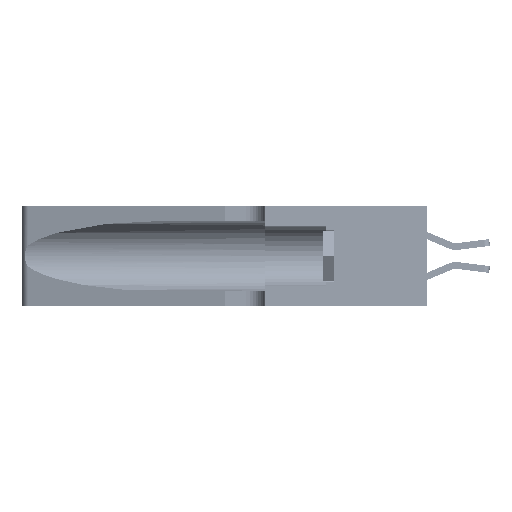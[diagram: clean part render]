
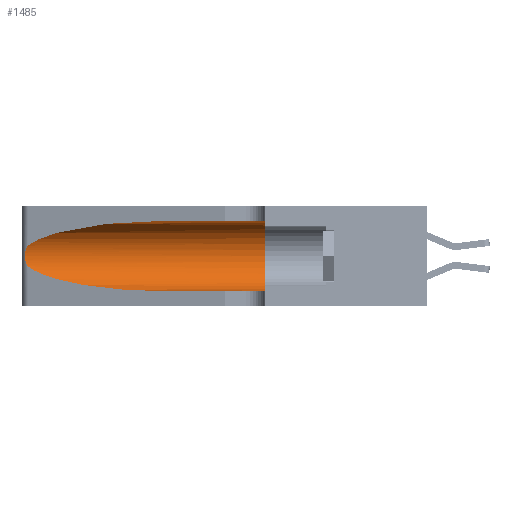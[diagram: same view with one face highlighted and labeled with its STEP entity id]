
A CAD part, left-side view. The second image highlights one B-rep face of the part: STEP entity #1485.
In plain terms, the highlighted cylindrical face has radius 3.308 mm (diameter 6.617 mm), a partial arc.
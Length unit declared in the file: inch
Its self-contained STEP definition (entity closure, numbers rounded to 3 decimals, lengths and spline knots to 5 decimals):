
#673 = ORIENTED_EDGE ( 'NONE', *, *, #36056, .T. ) ;
#773 = EDGE_LOOP ( 'NONE', ( #33767, #15607, #46806, #673, #40579, #41703 ) ) ;
#1485 = ADVANCED_FACE ( 'NONE', ( #13631 ), #41442, .F. ) ;
#1760 = DIRECTION ( 'NONE',  ( 0., -1., 0. ) ) ;
#2161 = VERTEX_POINT ( 'NONE', #34714 ) ;
#2343 = CARTESIAN_POINT ( 'NONE',  ( 0.18966, 0.96281, 0.31525 ) ) ;
#3633 = CARTESIAN_POINT ( 'NONE',  ( 0.25787, 1.23484, 0.2124 ) ) ;
#4534 = CARTESIAN_POINT ( 'NONE',  ( 0.25487, 1.22718, 0.14631 ) ) ;
#4576 = VERTEX_POINT ( 'NONE', #5747 ) ;
#5747 = CARTESIAN_POINT ( 'NONE',  ( 0.25487, 1.22718, 0.14631 ) ) ;
#7349 = CARTESIAN_POINT ( 'NONE',  ( 0.26018, 1.23835, 0.19895 ) ) ;
#8048 = CARTESIAN_POINT ( 'NONE',  ( 0.1305, 0.35, 0.05475 ) ) ;
#8570 = CARTESIAN_POINT ( 'NONE',  ( 0.25487, 1.22718, 0.22369 ) ) ;
#9151 = CARTESIAN_POINT ( 'NONE',  ( 0.1305, 1.61858, 0.185 ) ) ;
#10174 = EDGE_CURVE ( 'NONE', #12046, #4576, #31146, .T. ) ;
#10722 =( BOUNDED_CURVE ( )  B_SPLINE_CURVE ( 3, ( #4534, #33698, #11895, #37339 ),
 .UNSPECIFIED., .F., .T. ) 
 B_SPLINE_CURVE_WITH_KNOTS ( ( 4, 4 ),
 ( 3.44316, 4.71239 ),
 .UNSPECIFIED. ) 
 CURVE ( )  GEOMETRIC_REPRESENTATION_ITEM ( )  RATIONAL_B_SPLINE_CURVE ( ( 1., 0.87, 0.87, 1. ) ) 
 REPRESENTATION_ITEM ( '' )  );
#11016 = CARTESIAN_POINT ( 'NONE',  ( 0.26075, 1.23896, 0.178 ) ) ;
#11130 = CARTESIAN_POINT ( 'NONE',  ( 0.1305, 1.61858, 0.05475 ) ) ;
#11132 = AXIS2_PLACEMENT_3D ( 'NONE', #9151, #1760, #34617 ) ;
#11193 = DIRECTION ( 'NONE',  ( 0., -1., 0. ) ) ;
#11451 = AXIS2_PLACEMENT_3D ( 'NONE', #42541, #20803, #46184 ) ;
#11895 = CARTESIAN_POINT ( 'NONE',  ( 0.18966, 0.96281, 0.05475 ) ) ;
#12046 = VERTEX_POINT ( 'NONE', #8570 ) ;
#12978 = CARTESIAN_POINT ( 'NONE',  ( 0.1305, 0.72297, 0.31525 ) ) ;
#13415 = CARTESIAN_POINT ( 'NONE',  ( 0.25487, 1.22718, 0.22369 ) ) ;
#13631 = FACE_OUTER_BOUND ( 'NONE', #773, .T. ) ;
#14721 = CARTESIAN_POINT ( 'NONE',  ( 0.25856, 1.23593, 0.16098 ) ) ;
#15607 = ORIENTED_EDGE ( 'NONE', *, *, #10174, .T. ) ;
#18196 = CARTESIAN_POINT ( 'NONE',  ( 0.25487, 1.22718, 0.22369 ) ) ;
#18344 = CARTESIAN_POINT ( 'NONE',  ( 0.25639, 1.23186, 0.15144 ) ) ;
#20803 = DIRECTION ( 'NONE',  ( 0., 1., 0. ) ) ;
#21491 = CARTESIAN_POINT ( 'NONE',  ( 0.1305, 0.72297, 0.05475 ) ) ;
#22017 = CARTESIAN_POINT ( 'NONE',  ( 0.25487, 1.22718, 0.14631 ) ) ;
#25516 = CARTESIAN_POINT ( 'NONE',  ( 0.25639, 1.23184, 0.21858 ) ) ;
#26188 = VECTOR ( 'NONE', #11193, 39.37008 ) ;
#27868 = CARTESIAN_POINT ( 'NONE',  ( 0.1305, 0.72297, 0.31525 ) ) ;
#27886 = VERTEX_POINT ( 'NONE', #21491 ) ;
#28393 = EDGE_CURVE ( 'NONE', #2161, #38940, #32527, .T. ) ;
#29145 = CARTESIAN_POINT ( 'NONE',  ( 0.25854, 1.2359, 0.20912 ) ) ;
#31146 = B_SPLINE_CURVE_WITH_KNOTS ( 'NONE', 3,
 ( #18196, #36307, #25516, #3633, #29145, #7349, #32823, #11016, #36464, #14721, #40090, #18344, #43733, #22017 ),
 .UNSPECIFIED., .F., .F.,
 ( 4, 2, 2, 2, 2, 2, 4 ),
 ( 0., 0.00027, 0.00053, 0.00107, 0.0016, 0.00187, 0.00214 ),
 .UNSPECIFIED. ) ;
#31334 = VERTEX_POINT ( 'NONE', #12978 ) ;
#32527 = CIRCLE ( 'NONE', #11451, 0.13025 ) ;
#32615 =( BOUNDED_CURVE ( )  B_SPLINE_CURVE ( 3, ( #27868, #2343, #35198, #13415 ),
 .UNSPECIFIED., .F., .F. ) 
 B_SPLINE_CURVE_WITH_KNOTS ( ( 4, 4 ),
 ( 1.5708, 2.84003 ),
 .UNSPECIFIED. ) 
 CURVE ( )  GEOMETRIC_REPRESENTATION_ITEM ( )  RATIONAL_B_SPLINE_CURVE ( ( 1., 0.87, 0.87, 1. ) ) 
 REPRESENTATION_ITEM ( '' )  );
#32823 = CARTESIAN_POINT ( 'NONE',  ( 0.26075, 1.23896, 0.19203 ) ) ;
#32937 = DIRECTION ( 'NONE',  ( 0., -1., 0. ) ) ;
#32992 = CARTESIAN_POINT ( 'NONE',  ( 0.1305, 1.61858, 0.31525 ) ) ;
#33698 = CARTESIAN_POINT ( 'NONE',  ( 0.2373, 1.15595, 0.08982 ) ) ;
#33767 = ORIENTED_EDGE ( 'NONE', *, *, #42704, .T. ) ;
#34068 = VECTOR ( 'NONE', #32937, 39.37008 ) ;
#34617 = DIRECTION ( 'NONE',  ( 0., 0., -1. ) ) ;
#34714 = CARTESIAN_POINT ( 'NONE',  ( 0.1305, 0.35, 0.31525 ) ) ;
#35198 = CARTESIAN_POINT ( 'NONE',  ( 0.2373, 1.15595, 0.28018 ) ) ;
#35220 = LINE ( 'NONE', #11130, #34068 ) ;
#35364 = EDGE_CURVE ( 'NONE', #31334, #2161, #44345, .T. ) ;
#36056 = EDGE_CURVE ( 'NONE', #27886, #38940, #35220, .T. ) ;
#36307 = CARTESIAN_POINT ( 'NONE',  ( 0.25555, 1.22994, 0.2215 ) ) ;
#36353 = EDGE_CURVE ( 'NONE', #4576, #27886, #10722, .T. ) ;
#36464 = CARTESIAN_POINT ( 'NONE',  ( 0.26017, 1.23833, 0.17102 ) ) ;
#37339 = CARTESIAN_POINT ( 'NONE',  ( 0.1305, 0.72297, 0.05475 ) ) ;
#38940 = VERTEX_POINT ( 'NONE', #8048 ) ;
#40090 = CARTESIAN_POINT ( 'NONE',  ( 0.25789, 1.23486, 0.15765 ) ) ;
#40579 = ORIENTED_EDGE ( 'NONE', *, *, #28393, .F. ) ;
#41442 = CYLINDRICAL_SURFACE ( 'NONE', #11132, 0.13025 ) ;
#41703 = ORIENTED_EDGE ( 'NONE', *, *, #35364, .F. ) ;
#42541 = CARTESIAN_POINT ( 'NONE',  ( 0.1305, 0.35, 0.185 ) ) ;
#42704 = EDGE_CURVE ( 'NONE', #31334, #12046, #32615, .T. ) ;
#43733 = CARTESIAN_POINT ( 'NONE',  ( 0.25555, 1.22993, 0.14849 ) ) ;
#44345 = LINE ( 'NONE', #32992, #26188 ) ;
#46184 = DIRECTION ( 'NONE',  ( 0., 0., 1. ) ) ;
#46806 = ORIENTED_EDGE ( 'NONE', *, *, #36353, .T. ) ;
